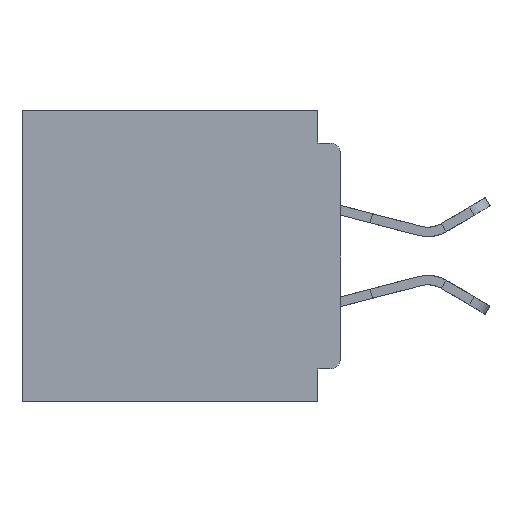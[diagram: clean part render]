
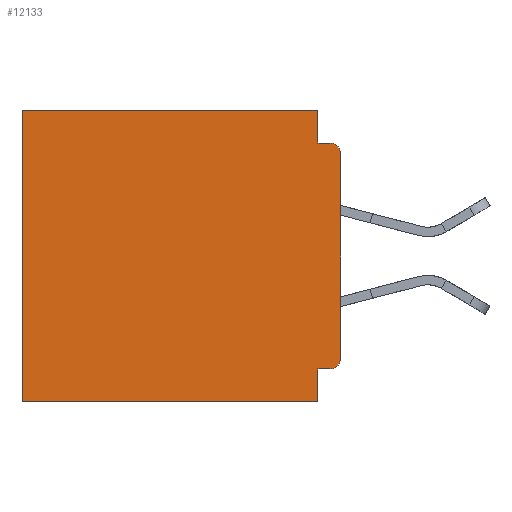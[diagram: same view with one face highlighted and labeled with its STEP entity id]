
A CAD part, left-side view. The second image highlights one B-rep face of the part: STEP entity #12133.
In plain terms, the highlighted planar face has unit normal (-1, 0, 0).
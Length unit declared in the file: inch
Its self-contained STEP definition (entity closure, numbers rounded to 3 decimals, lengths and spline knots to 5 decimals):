
#66 = LINE ( 'NONE', #23175, #18659 ) ;
#342 = CARTESIAN_POINT ( 'NONE',  ( 0.3, 0.437, 0. ) ) ;
#1054 = ORIENTED_EDGE ( 'NONE', *, *, #44980, .F. ) ;
#1810 = VERTEX_POINT ( 'NONE', #22947 ) ;
#2565 = CARTESIAN_POINT ( 'NONE',  ( 0.3, 0.437, -0.4 ) ) ;
#3211 = EDGE_CURVE ( 'NONE', #28098, #15745, #43805, .T. ) ;
#4667 = AXIS2_PLACEMENT_3D ( 'NONE', #27163, #5078, #30836 ) ;
#5078 = DIRECTION ( 'NONE',  ( 1., 0., 0. ) ) ;
#5738 = VECTOR ( 'NONE', #33127, 39.37008 ) ;
#6232 = VERTEX_POINT ( 'NONE', #23103 ) ;
#7806 = CARTESIAN_POINT ( 'NONE',  ( 0.3, 0., -0.06 ) ) ;
#8573 = CARTESIAN_POINT ( 'NONE',  ( 0.3, 0.031, -0.4 ) ) ;
#9196 = EDGE_CURVE ( 'NONE', #23759, #23790, #33042, .T. ) ;
#10329 = EDGE_CURVE ( 'NONE', #1810, #34091, #42171, .T. ) ;
#11477 = VERTEX_POINT ( 'NONE', #30740 ) ;
#12086 = EDGE_CURVE ( 'NONE', #30986, #14756, #66, .T. ) ;
#12133 = ADVANCED_FACE ( 'NONE', ( #16327 ), #27008, .F. ) ;
#12915 = DIRECTION ( 'NONE',  ( -1., 0., 0. ) ) ;
#13018 = VECTOR ( 'NONE', #44204, 39.37008 ) ;
#13082 = DIRECTION ( 'NONE',  ( -1., 0., 0. ) ) ;
#13405 = EDGE_LOOP ( 'NONE', ( #20536, #38295, #39109, #23001, #20098, #26911, #31209, #13521, #1054, #29506 ) ) ;
#13435 = VECTOR ( 'NONE', #46974, 39.37008 ) ;
#13521 = ORIENTED_EDGE ( 'NONE', *, *, #9196, .F. ) ;
#14297 = CARTESIAN_POINT ( 'NONE',  ( 0.3, 0., 0. ) ) ;
#14756 = VERTEX_POINT ( 'NONE', #2565 ) ;
#15224 = VECTOR ( 'NONE', #42666, 39.37008 ) ;
#15745 = VERTEX_POINT ( 'NONE', #45202 ) ;
#15933 = DIRECTION ( 'NONE',  ( 0., 0., -1. ) ) ;
#16327 = FACE_OUTER_BOUND ( 'NONE', #13405, .T. ) ;
#17257 = VECTOR ( 'NONE', #18014, 39.37008 ) ;
#18014 = DIRECTION ( 'NONE',  ( 0., 1., 0. ) ) ;
#18659 = VECTOR ( 'NONE', #15933, 39.37008 ) ;
#19588 = EDGE_CURVE ( 'NONE', #11477, #15745, #42031, .T. ) ;
#20098 = ORIENTED_EDGE ( 'NONE', *, *, #40308, .T. ) ;
#20536 = ORIENTED_EDGE ( 'NONE', *, *, #3211, .F. ) ;
#22915 = CARTESIAN_POINT ( 'NONE',  ( 0.3, 0.031, -0.355 ) ) ;
#22947 = CARTESIAN_POINT ( 'NONE',  ( 0.3, 0.031, 0. ) ) ;
#23001 = ORIENTED_EDGE ( 'NONE', *, *, #10329, .F. ) ;
#23103 = CARTESIAN_POINT ( 'NONE',  ( 0.3, 0.015, -0.045 ) ) ;
#23175 = CARTESIAN_POINT ( 'NONE',  ( 0.3, 0.437, -0.4 ) ) ;
#23316 = VECTOR ( 'NONE', #38615, 39.37008 ) ;
#23759 = VERTEX_POINT ( 'NONE', #22915 ) ;
#23790 = VERTEX_POINT ( 'NONE', #8573 ) ;
#24094 = EDGE_CURVE ( 'NONE', #23790, #14756, #42795, .T. ) ;
#25030 = LINE ( 'NONE', #39120, #15224 ) ;
#26911 = ORIENTED_EDGE ( 'NONE', *, *, #12086, .T. ) ;
#27008 = PLANE ( 'NONE',  #4667 ) ;
#27163 = CARTESIAN_POINT ( 'NONE',  ( 0.3, 0., -0.4 ) ) ;
#28098 = VERTEX_POINT ( 'NONE', #7806 ) ;
#29506 = ORIENTED_EDGE ( 'NONE', *, *, #19588, .T. ) ;
#30740 = CARTESIAN_POINT ( 'NONE',  ( 0.3, 0.015, -0.355 ) ) ;
#30836 = DIRECTION ( 'NONE',  ( 0., 0., -1. ) ) ;
#30924 = CARTESIAN_POINT ( 'NONE',  ( 0.3, 0.031, -0.045 ) ) ;
#30986 = VERTEX_POINT ( 'NONE', #342 ) ;
#31184 = CARTESIAN_POINT ( 'NONE',  ( 0.3, 0.031, -0.4 ) ) ;
#31209 = ORIENTED_EDGE ( 'NONE', *, *, #24094, .F. ) ;
#32317 = CARTESIAN_POINT ( 'NONE',  ( 0.3, 0., -0.4 ) ) ;
#32340 = VECTOR ( 'NONE', #41571, 39.37008 ) ;
#32535 = LINE ( 'NONE', #33052, #13018 ) ;
#33042 = LINE ( 'NONE', #31184, #23316 ) ;
#33052 = CARTESIAN_POINT ( 'NONE',  ( 0.3, 0., -0.045 ) ) ;
#33064 = CARTESIAN_POINT ( 'NONE',  ( 0.3, 0., -0.4 ) ) ;
#33127 = DIRECTION ( 'NONE',  ( 0., 0., -1. ) ) ;
#34091 = VERTEX_POINT ( 'NONE', #30924 ) ;
#34901 = CARTESIAN_POINT ( 'NONE',  ( 0.3, 0.015, -0.34 ) ) ;
#35074 = CARTESIAN_POINT ( 'NONE',  ( 0.3, 0.015, -0.06 ) ) ;
#35613 = LINE ( 'NONE', #14297, #17257 ) ;
#38295 = ORIENTED_EDGE ( 'NONE', *, *, #44925, .T. ) ;
#38615 = DIRECTION ( 'NONE',  ( 0., 0., -1. ) ) ;
#38628 = DIRECTION ( 'NONE',  ( 0., 0., -1. ) ) ;
#38801 = DIRECTION ( 'NONE',  ( 0., 0., -1. ) ) ;
#39109 = ORIENTED_EDGE ( 'NONE', *, *, #44120, .F. ) ;
#39120 = CARTESIAN_POINT ( 'NONE',  ( 0.3, 0., -0.355 ) ) ;
#40308 = EDGE_CURVE ( 'NONE', #1810, #30986, #35613, .T. ) ;
#41408 = CARTESIAN_POINT ( 'NONE',  ( 0.3, 0.031, 0. ) ) ;
#41571 = DIRECTION ( 'NONE',  ( 0., 0., -1. ) ) ;
#42031 = CIRCLE ( 'NONE', #46838, 0.015 ) ;
#42171 = LINE ( 'NONE', #41408, #32340 ) ;
#42666 = DIRECTION ( 'NONE',  ( 0., 1., 0. ) ) ;
#42795 = LINE ( 'NONE', #32317, #13435 ) ;
#43728 = AXIS2_PLACEMENT_3D ( 'NONE', #35074, #13082, #38801 ) ;
#43805 = LINE ( 'NONE', #33064, #5738 ) ;
#44120 = EDGE_CURVE ( 'NONE', #34091, #6232, #32535, .T. ) ;
#44204 = DIRECTION ( 'NONE',  ( 0., -1., 0. ) ) ;
#44925 = EDGE_CURVE ( 'NONE', #28098, #6232, #45733, .T. ) ;
#44980 = EDGE_CURVE ( 'NONE', #11477, #23759, #25030, .T. ) ;
#45202 = CARTESIAN_POINT ( 'NONE',  ( 0.3, 0., -0.34 ) ) ;
#45733 = CIRCLE ( 'NONE', #43728, 0.015 ) ;
#46838 = AXIS2_PLACEMENT_3D ( 'NONE', #34901, #12915, #38628 ) ;
#46974 = DIRECTION ( 'NONE',  ( 0., 1., 0. ) ) ;
